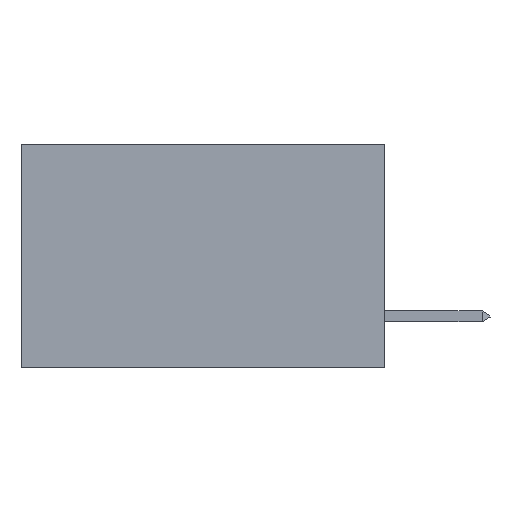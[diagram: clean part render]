
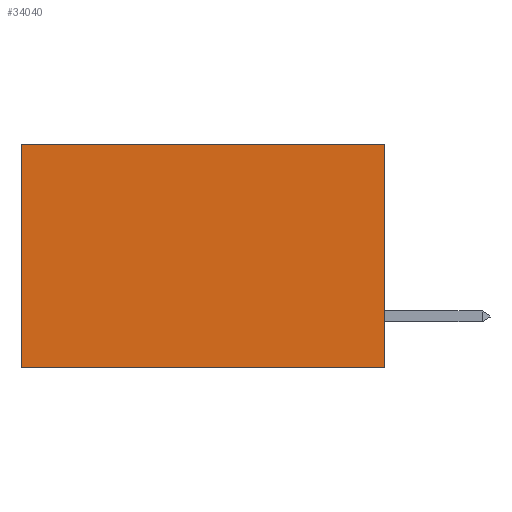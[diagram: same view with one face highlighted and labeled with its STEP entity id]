
A CAD part, left-side view. The second image highlights one B-rep face of the part: STEP entity #34040.
In plain terms, the highlighted planar face has unit normal (-1, 0, 0).
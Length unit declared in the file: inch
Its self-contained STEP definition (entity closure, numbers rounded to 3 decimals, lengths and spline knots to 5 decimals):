
#241 = ORIENTED_EDGE ( 'NONE', *, *, #23877, .F. ) ;
#1373 = EDGE_LOOP ( 'NONE', ( #16465, #241, #38454, #28146 ) ) ;
#3360 = CARTESIAN_POINT ( 'NONE',  ( 0.2875, 0., 0. ) ) ;
#3936 = LINE ( 'NONE', #3360, #38739 ) ;
#5050 = CARTESIAN_POINT ( 'NONE',  ( 0.2875, 0.6, 0. ) ) ;
#6268 = VERTEX_POINT ( 'NONE', #5050 ) ;
#6482 = VECTOR ( 'NONE', #8753, 39.37008 ) ;
#8666 = FACE_OUTER_BOUND ( 'NONE', #1373, .T. ) ;
#8753 = DIRECTION ( 'NONE',  ( 0., 1., 0. ) ) ;
#9625 = PLANE ( 'NONE',  #26038 ) ;
#11412 = CARTESIAN_POINT ( 'NONE',  ( 0.2875, 0.6, -0.37 ) ) ;
#13577 = LINE ( 'NONE', #42995, #6482 ) ;
#13726 = DIRECTION ( 'NONE',  ( 0., 0., -1. ) ) ;
#14203 = VECTOR ( 'NONE', #20592, 39.37008 ) ;
#16465 = ORIENTED_EDGE ( 'NONE', *, *, #23232, .T. ) ;
#18891 = LINE ( 'NONE', #46860, #14203 ) ;
#20592 = DIRECTION ( 'NONE',  ( 0., 0., -1. ) ) ;
#21932 = DIRECTION ( 'NONE',  ( 0., 0., -1. ) ) ;
#22078 = CARTESIAN_POINT ( 'NONE',  ( 0.2875, 0., 0. ) ) ;
#22920 = VECTOR ( 'NONE', #21932, 39.37008 ) ;
#23232 = EDGE_CURVE ( 'NONE', #6268, #39740, #18891, .T. ) ;
#23877 = EDGE_CURVE ( 'NONE', #39631, #39740, #13577, .T. ) ;
#24903 = VERTEX_POINT ( 'NONE', #34301 ) ;
#26038 = AXIS2_PLACEMENT_3D ( 'NONE', #43723, #36260, #13726 ) ;
#26443 = LINE ( 'NONE', #22078, #22920 ) ;
#28146 = ORIENTED_EDGE ( 'NONE', *, *, #30089, .T. ) ;
#29686 = DIRECTION ( 'NONE',  ( 0., 1., 0. ) ) ;
#30089 = EDGE_CURVE ( 'NONE', #24903, #6268, #3936, .T. ) ;
#32419 = EDGE_CURVE ( 'NONE', #24903, #39631, #26443, .T. ) ;
#34040 = ADVANCED_FACE ( 'NONE', ( #8666 ), #9625, .F. ) ;
#34301 = CARTESIAN_POINT ( 'NONE',  ( 0.2875, 0., 0. ) ) ;
#36260 = DIRECTION ( 'NONE',  ( 1., 0., 0. ) ) ;
#38454 = ORIENTED_EDGE ( 'NONE', *, *, #32419, .F. ) ;
#38739 = VECTOR ( 'NONE', #29686, 39.37008 ) ;
#39631 = VERTEX_POINT ( 'NONE', #48041 ) ;
#39740 = VERTEX_POINT ( 'NONE', #11412 ) ;
#42995 = CARTESIAN_POINT ( 'NONE',  ( 0.2875, 0., -0.37 ) ) ;
#43723 = CARTESIAN_POINT ( 'NONE',  ( 0.2875, 0., 0. ) ) ;
#46860 = CARTESIAN_POINT ( 'NONE',  ( 0.2875, 0.6, 0. ) ) ;
#48041 = CARTESIAN_POINT ( 'NONE',  ( 0.2875, 0., -0.37 ) ) ;
